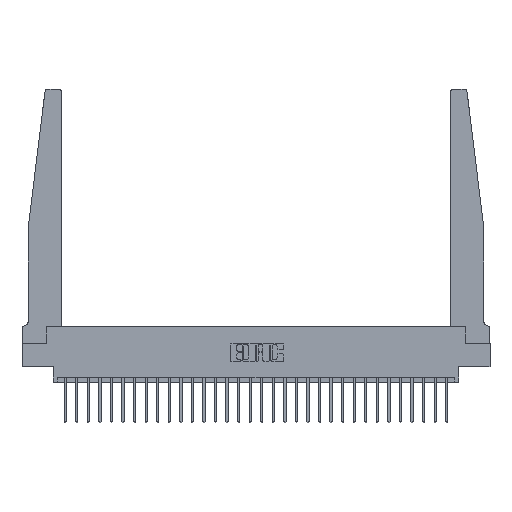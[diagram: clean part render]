
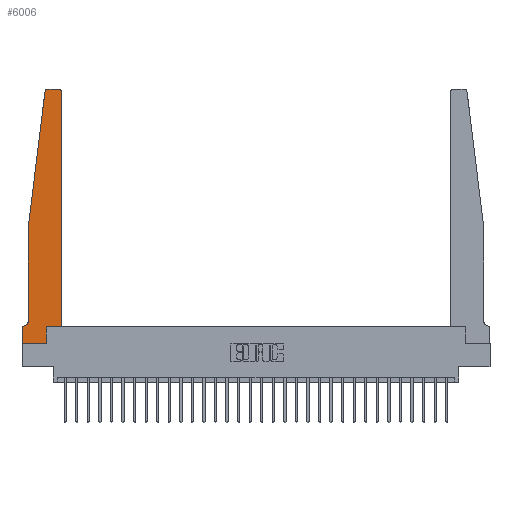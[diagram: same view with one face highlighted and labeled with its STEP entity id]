
A CAD part, top view. The second image highlights one B-rep face of the part: STEP entity #6006.
In plain terms, the highlighted planar face has unit normal (0, 0, 1).
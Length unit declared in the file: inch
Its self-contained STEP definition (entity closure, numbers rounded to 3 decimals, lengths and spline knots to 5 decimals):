
#395 = VERTEX_POINT ( 'NONE', #14037 ) ;
#530 = CARTESIAN_POINT ( 'NONE',  ( 0.015, 0.1875, 0.37 ) ) ;
#547 = LINE ( 'NONE', #9047, #5092 ) ;
#744 = DIRECTION ( 'NONE',  ( 0., 0., 1. ) ) ;
#920 = DIRECTION ( 'NONE',  ( -0.122, -0.992, 0. ) ) ;
#985 = VERTEX_POINT ( 'NONE', #530 ) ;
#1114 = EDGE_CURVE ( 'NONE', #9413, #13783, #14676, .T. ) ;
#1502 = EDGE_CURVE ( 'NONE', #14418, #2696, #26776, .T. ) ;
#1513 = VERTEX_POINT ( 'NONE', #5147 ) ;
#1592 = EDGE_CURVE ( 'NONE', #13783, #22242, #25444, .T. ) ;
#1672 = LINE ( 'NONE', #6507, #24171 ) ;
#1755 = CARTESIAN_POINT ( 'NONE',  ( 0., 0., 0.37 ) ) ;
#1986 = LINE ( 'NONE', #11552, #2677 ) ;
#2051 = CARTESIAN_POINT ( 'NONE',  ( 0.425, 0.18, 0.37 ) ) ;
#2677 = VECTOR ( 'NONE', #9248, 39.37008 ) ;
#2696 = VERTEX_POINT ( 'NONE', #9365 ) ;
#3259 = CIRCLE ( 'NONE', #20736, 0.03 ) ;
#3294 = VERTEX_POINT ( 'NONE', #17996 ) ;
#3357 = EDGE_CURVE ( 'NONE', #13006, #9413, #3259, .T. ) ;
#4089 = ORIENTED_EDGE ( 'NONE', *, *, #3357, .T. ) ;
#4885 = DIRECTION ( 'NONE',  ( 1., 0., 0. ) ) ;
#4901 = VERTEX_POINT ( 'NONE', #13919 ) ;
#5092 = VECTOR ( 'NONE', #13250, 39.37008 ) ;
#5147 = CARTESIAN_POINT ( 'NONE',  ( 0.425, 0.18, 0.37 ) ) ;
#5633 = VECTOR ( 'NONE', #25451, 39.37008 ) ;
#5953 = DIRECTION ( 'NONE',  ( 0., 0., 1. ) ) ;
#6006 = ADVANCED_FACE ( 'NONE', ( #15738 ), #15727, .T. ) ;
#6147 = DIRECTION ( 'NONE',  ( 0., 0., -1. ) ) ;
#6507 = CARTESIAN_POINT ( 'NONE',  ( 0.25, 2.75, 0.37 ) ) ;
#6727 = ORIENTED_EDGE ( 'NONE', *, *, #7631, .T. ) ;
#7324 = CARTESIAN_POINT ( 'NONE',  ( 0., 0., 0.37 ) ) ;
#7631 = EDGE_CURVE ( 'NONE', #9169, #395, #25004, .T. ) ;
#7878 = LINE ( 'NONE', #15680, #24500 ) ;
#9047 = CARTESIAN_POINT ( 'NONE',  ( 0.425, 0.18, 0.37 ) ) ;
#9169 = VERTEX_POINT ( 'NONE', #17496 ) ;
#9248 = DIRECTION ( 'NONE',  ( 0., -1., 0. ) ) ;
#9365 = CARTESIAN_POINT ( 'NONE',  ( 0.2605, 0., 0.37 ) ) ;
#9413 = VERTEX_POINT ( 'NONE', #27359 ) ;
#9533 = ORIENTED_EDGE ( 'NONE', *, *, #21758, .T. ) ;
#10061 = ORIENTED_EDGE ( 'NONE', *, *, #10916, .T. ) ;
#10667 = CIRCLE ( 'NONE', #25354, 0.05 ) ;
#10916 = EDGE_CURVE ( 'NONE', #22242, #985, #10667, .T. ) ;
#10918 = DIRECTION ( 'NONE',  ( -1., 0., 0. ) ) ;
#10974 = ORIENTED_EDGE ( 'NONE', *, *, #26083, .T. ) ;
#11552 = CARTESIAN_POINT ( 'NONE',  ( 0., 0., 0.37 ) ) ;
#11764 = EDGE_CURVE ( 'NONE', #1513, #9169, #11982, .T. ) ;
#11982 = LINE ( 'NONE', #2051, #17743 ) ;
#12319 = ORIENTED_EDGE ( 'NONE', *, *, #12490, .T. ) ;
#12490 = EDGE_CURVE ( 'NONE', #3294, #1513, #547, .T. ) ;
#13001 = DIRECTION ( 'NONE',  ( 0., 1., 0. ) ) ;
#13006 = VERTEX_POINT ( 'NONE', #17015 ) ;
#13250 = DIRECTION ( 'NONE',  ( 1., 0., 0. ) ) ;
#13535 = DIRECTION ( 'NONE',  ( -1., 0., 0. ) ) ;
#13580 = CARTESIAN_POINT ( 'NONE',  ( 0., 0.1875, 0.37 ) ) ;
#13783 = VERTEX_POINT ( 'NONE', #14357 ) ;
#13919 = CARTESIAN_POINT ( 'NONE',  ( 0., 0.1875, 0.37 ) ) ;
#13928 = CARTESIAN_POINT ( 'NONE',  ( 0.27653, 2.72, 0.37 ) ) ;
#14037 = CARTESIAN_POINT ( 'NONE',  ( 0.395, 2.75, 0.37 ) ) ;
#14357 = CARTESIAN_POINT ( 'NONE',  ( 0.065, 1.25, 0.37 ) ) ;
#14418 = VERTEX_POINT ( 'NONE', #1755 ) ;
#14676 = LINE ( 'NONE', #24839, #25466 ) ;
#14993 = AXIS2_PLACEMENT_3D ( 'NONE', #13580, #17928, #4885 ) ;
#15086 = ORIENTED_EDGE ( 'NONE', *, *, #11764, .T. ) ;
#15513 = ORIENTED_EDGE ( 'NONE', *, *, #1114, .T. ) ;
#15680 = CARTESIAN_POINT ( 'NONE',  ( 0.065, 0.1875, 0.37 ) ) ;
#15727 = PLANE ( 'NONE',  #14993 ) ;
#15738 = FACE_OUTER_BOUND ( 'NONE', #25115, .T. ) ;
#15929 = ORIENTED_EDGE ( 'NONE', *, *, #22495, .T. ) ;
#16079 = DIRECTION ( 'NONE',  ( 1., 0., 0. ) ) ;
#17015 = CARTESIAN_POINT ( 'NONE',  ( 0.27653, 2.75, 0.37 ) ) ;
#17496 = CARTESIAN_POINT ( 'NONE',  ( 0.425, 2.72, 0.37 ) ) ;
#17743 = VECTOR ( 'NONE', #13001, 39.37008 ) ;
#17928 = DIRECTION ( 'NONE',  ( 0., 0., 1. ) ) ;
#17996 = CARTESIAN_POINT ( 'NONE',  ( 0.2605, 0.18, 0.37 ) ) ;
#18028 = EDGE_CURVE ( 'NONE', #985, #4901, #7878, .T. ) ;
#18357 = ORIENTED_EDGE ( 'NONE', *, *, #1502, .T. ) ;
#18850 = CARTESIAN_POINT ( 'NONE',  ( 0.065, 1.25, 0.37 ) ) ;
#18997 = CARTESIAN_POINT ( 'NONE',  ( 0.395, 2.72, 0.37 ) ) ;
#19045 = VECTOR ( 'NONE', #20997, 39.37008 ) ;
#19207 = CARTESIAN_POINT ( 'NONE',  ( 0.015, 0.2375, 0.37 ) ) ;
#20072 = AXIS2_PLACEMENT_3D ( 'NONE', #18997, #5953, #21150 ) ;
#20736 = AXIS2_PLACEMENT_3D ( 'NONE', #13928, #744, #16079 ) ;
#20997 = DIRECTION ( 'NONE',  ( 0., -1., 0. ) ) ;
#21150 = DIRECTION ( 'NONE',  ( 1., 0., 0. ) ) ;
#21356 = DIRECTION ( 'NONE',  ( -1., 0., 0. ) ) ;
#21738 = VECTOR ( 'NONE', #22509, 39.37008 ) ;
#21758 = EDGE_CURVE ( 'NONE', #395, #13006, #1672, .T. ) ;
#22242 = VERTEX_POINT ( 'NONE', #25630 ) ;
#22495 = EDGE_CURVE ( 'NONE', #4901, #14418, #1986, .T. ) ;
#22509 = DIRECTION ( 'NONE',  ( 1., 0., 0. ) ) ;
#22945 = LINE ( 'NONE', #23270, #5633 ) ;
#23270 = CARTESIAN_POINT ( 'NONE',  ( 0.2605, 0.18, 0.37 ) ) ;
#24171 = VECTOR ( 'NONE', #10918, 39.37008 ) ;
#24500 = VECTOR ( 'NONE', #13535, 39.37008 ) ;
#24839 = CARTESIAN_POINT ( 'NONE',  ( 0.065, 1.25, 0.37 ) ) ;
#25004 = CIRCLE ( 'NONE', #20072, 0.03 ) ;
#25115 = EDGE_LOOP ( 'NONE', ( #9533, #4089, #15513, #27616, #10061, #28056, #15929, #18357, #10974, #12319, #15086, #6727 ) ) ;
#25354 = AXIS2_PLACEMENT_3D ( 'NONE', #19207, #6147, #21356 ) ;
#25444 = LINE ( 'NONE', #18850, #19045 ) ;
#25451 = DIRECTION ( 'NONE',  ( 0., 1., 0. ) ) ;
#25466 = VECTOR ( 'NONE', #920, 39.37008 ) ;
#25630 = CARTESIAN_POINT ( 'NONE',  ( 0.065, 0.2375, 0.37 ) ) ;
#26083 = EDGE_CURVE ( 'NONE', #2696, #3294, #22945, .T. ) ;
#26776 = LINE ( 'NONE', #7324, #21738 ) ;
#27359 = CARTESIAN_POINT ( 'NONE',  ( 0.24675, 2.72367, 0.37 ) ) ;
#27616 = ORIENTED_EDGE ( 'NONE', *, *, #1592, .T. ) ;
#28056 = ORIENTED_EDGE ( 'NONE', *, *, #18028, .T. ) ;
